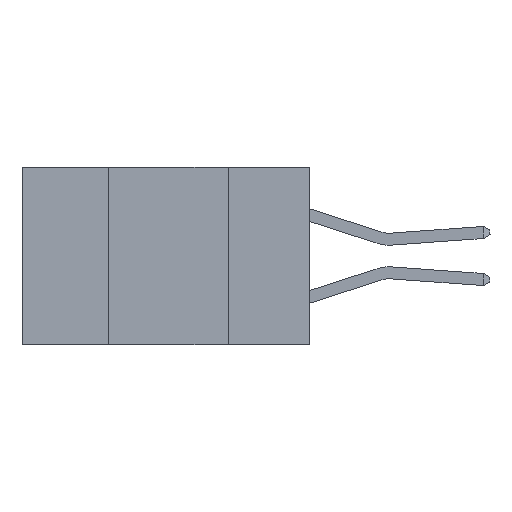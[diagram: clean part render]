
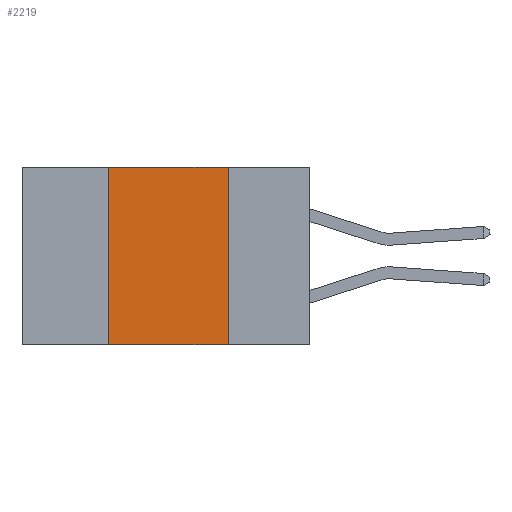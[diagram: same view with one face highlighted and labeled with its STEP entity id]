
A CAD part, left-side view. The second image highlights one B-rep face of the part: STEP entity #2219.
In plain terms, the highlighted planar face has unit normal (-1, 0, 0).
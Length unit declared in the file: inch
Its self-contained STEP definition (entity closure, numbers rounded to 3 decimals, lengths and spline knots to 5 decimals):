
#109 = EDGE_CURVE ( 'NONE', #1475, #7897, #6282, .T. ) ;
#230 = VERTEX_POINT ( 'NONE', #4980 ) ;
#284 = CARTESIAN_POINT ( 'NONE',  ( 0., 0.17, -0.37 ) ) ;
#289 = VECTOR ( 'NONE', #3249, 39.37008 ) ;
#471 = CARTESIAN_POINT ( 'NONE',  ( 0., 0.17, 0. ) ) ;
#1398 = CARTESIAN_POINT ( 'NONE',  ( 0., 0.42, -0.37 ) ) ;
#1475 = VERTEX_POINT ( 'NONE', #471 ) ;
#1479 = LINE ( 'NONE', #1398, #4099 ) ;
#2219 = ADVANCED_FACE ( 'NONE', ( #12381 ), #3168, .F. ) ;
#2717 = DIRECTION ( 'NONE',  ( 0., 0., -1. ) ) ;
#2786 = DIRECTION ( 'NONE',  ( 1., 0., 0. ) ) ;
#2835 = CARTESIAN_POINT ( 'NONE',  ( 0., 0.42, -0.37 ) ) ;
#2897 = LINE ( 'NONE', #5222, #289 ) ;
#3168 = PLANE ( 'NONE',  #4768 ) ;
#3249 = DIRECTION ( 'NONE',  ( 0., -1., 0. ) ) ;
#4099 = VECTOR ( 'NONE', #8255, 39.37008 ) ;
#4230 = VECTOR ( 'NONE', #6683, 39.37008 ) ;
#4539 = LINE ( 'NONE', #11481, #4230 ) ;
#4768 = AXIS2_PLACEMENT_3D ( 'NONE', #5576, #2786, #2717 ) ;
#4980 = CARTESIAN_POINT ( 'NONE',  ( 0., 0.42, 0. ) ) ;
#5222 = CARTESIAN_POINT ( 'NONE',  ( 0., 0.6, -0.37 ) ) ;
#5313 = VERTEX_POINT ( 'NONE', #2835 ) ;
#5576 = CARTESIAN_POINT ( 'NONE',  ( 0., 0.6, 0. ) ) ;
#6282 = LINE ( 'NONE', #6335, #8593 ) ;
#6335 = CARTESIAN_POINT ( 'NONE',  ( 0., 0.17, -0.37 ) ) ;
#6683 = DIRECTION ( 'NONE',  ( 0., -1., 0. ) ) ;
#6733 = ORIENTED_EDGE ( 'NONE', *, *, #9548, .T. ) ;
#7253 = EDGE_LOOP ( 'NONE', ( #8303, #7739, #7707, #6733 ) ) ;
#7707 = ORIENTED_EDGE ( 'NONE', *, *, #11433, .F. ) ;
#7739 = ORIENTED_EDGE ( 'NONE', *, *, #12030, .F. ) ;
#7897 = VERTEX_POINT ( 'NONE', #284 ) ;
#8255 = DIRECTION ( 'NONE',  ( 0., 0., 1. ) ) ;
#8303 = ORIENTED_EDGE ( 'NONE', *, *, #109, .F. ) ;
#8593 = VECTOR ( 'NONE', #11314, 39.37008 ) ;
#9548 = EDGE_CURVE ( 'NONE', #5313, #7897, #2897, .T. ) ;
#11314 = DIRECTION ( 'NONE',  ( 0., 0., -1. ) ) ;
#11433 = EDGE_CURVE ( 'NONE', #5313, #230, #1479, .T. ) ;
#11481 = CARTESIAN_POINT ( 'NONE',  ( 0., 0.6, 0. ) ) ;
#12030 = EDGE_CURVE ( 'NONE', #230, #1475, #4539, .T. ) ;
#12381 = FACE_OUTER_BOUND ( 'NONE', #7253, .T. ) ;
